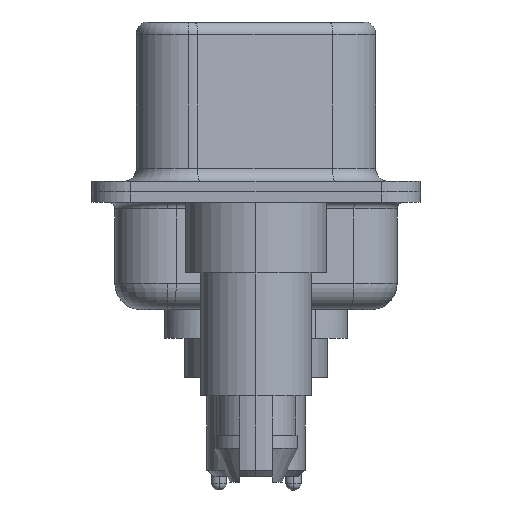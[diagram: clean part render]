
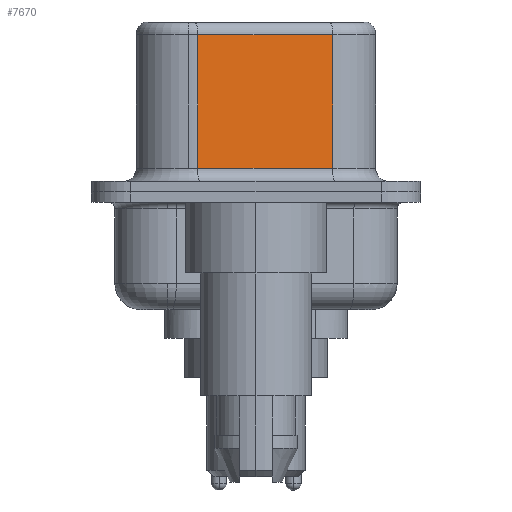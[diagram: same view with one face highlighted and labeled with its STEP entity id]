
A CAD part, left-side view. The second image highlights one B-rep face of the part: STEP entity #7670.
In plain terms, the highlighted planar face has unit normal (-0.985, -0.174, 0).
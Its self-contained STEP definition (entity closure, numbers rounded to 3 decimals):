
#516 = CARTESIAN_POINT ( 'NONE',  ( 4.585, -2.927, 6.02 ) ) ;
#1519 = CARTESIAN_POINT ( 'NONE',  ( 4.585, -2.927, 6.52 ) ) ;
#1742 = CARTESIAN_POINT ( 'NONE',  ( 3.675, 2.233, 0.9 ) ) ;
#2141 = VERTEX_POINT ( 'NONE', #1742 ) ;
#2231 = VECTOR ( 'NONE', #11079, 1000. ) ;
#2661 = EDGE_CURVE ( 'NONE', #8685, #17599, #2733, .T. ) ;
#2733 = LINE ( 'NONE', #1519, #2231 ) ;
#3239 = FACE_OUTER_BOUND ( 'NONE', #6486, .T. ) ;
#3518 = CARTESIAN_POINT ( 'NONE',  ( 4.585, -2.927, 0.9 ) ) ;
#4571 = LINE ( 'NONE', #516, #6771 ) ;
#5488 = CARTESIAN_POINT ( 'NONE',  ( 3.675, 2.233, 6.52 ) ) ;
#5516 = VECTOR ( 'NONE', #7365, 1000. ) ;
#6486 = EDGE_LOOP ( 'NONE', ( #19619, #17920, #17286, #11842 ) ) ;
#6771 = VECTOR ( 'NONE', #19457, 1000. ) ;
#7116 = CARTESIAN_POINT ( 'NONE',  ( 4.585, -2.927, 6.52 ) ) ;
#7365 = DIRECTION ( 'NONE',  ( 0.174, -0.985, 0. ) ) ;
#7670 = ADVANCED_FACE ( 'NONE', ( #3239 ), #16628, .F. ) ;
#8685 = VERTEX_POINT ( 'NONE', #17760 ) ;
#10237 = DIRECTION ( 'NONE',  ( 0.985, 0.174, 0. ) ) ;
#10254 = DIRECTION ( 'NONE',  ( 0., 0., -1. ) ) ;
#10282 = CARTESIAN_POINT ( 'NONE',  ( 3.675, 2.233, 6.02 ) ) ;
#10498 = LINE ( 'NONE', #15373, #5516 ) ;
#10962 = LINE ( 'NONE', #5488, #12956 ) ;
#11079 = DIRECTION ( 'NONE',  ( 0., 0., -1. ) ) ;
#11842 = ORIENTED_EDGE ( 'NONE', *, *, #17382, .T. ) ;
#12276 = AXIS2_PLACEMENT_3D ( 'NONE', #7116, #10237, #15189 ) ;
#12956 = VECTOR ( 'NONE', #10254, 1000. ) ;
#13030 = VERTEX_POINT ( 'NONE', #10282 ) ;
#15189 = DIRECTION ( 'NONE',  ( -0.174, 0.985, 0. ) ) ;
#15373 = CARTESIAN_POINT ( 'NONE',  ( 4.585, -2.927, 0.9 ) ) ;
#16479 = EDGE_CURVE ( 'NONE', #8685, #13030, #4571, .T. ) ;
#16628 = PLANE ( 'NONE',  #12276 ) ;
#17286 = ORIENTED_EDGE ( 'NONE', *, *, #17825, .T. ) ;
#17382 = EDGE_CURVE ( 'NONE', #2141, #17599, #10498, .T. ) ;
#17599 = VERTEX_POINT ( 'NONE', #3518 ) ;
#17760 = CARTESIAN_POINT ( 'NONE',  ( 4.585, -2.927, 6.02 ) ) ;
#17825 = EDGE_CURVE ( 'NONE', #13030, #2141, #10962, .T. ) ;
#17920 = ORIENTED_EDGE ( 'NONE', *, *, #16479, .T. ) ;
#19457 = DIRECTION ( 'NONE',  ( -0.174, 0.985, 0. ) ) ;
#19619 = ORIENTED_EDGE ( 'NONE', *, *, #2661, .F. ) ;
